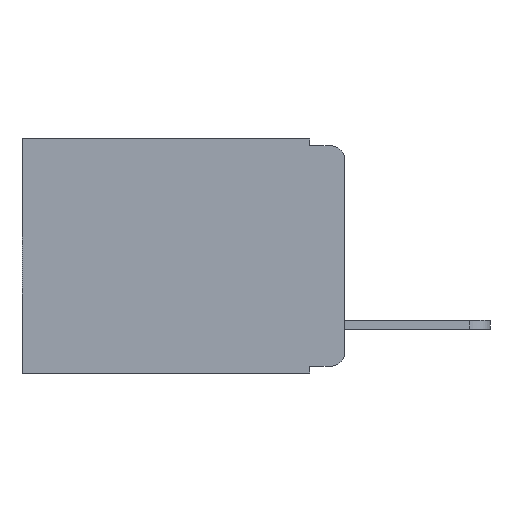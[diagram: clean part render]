
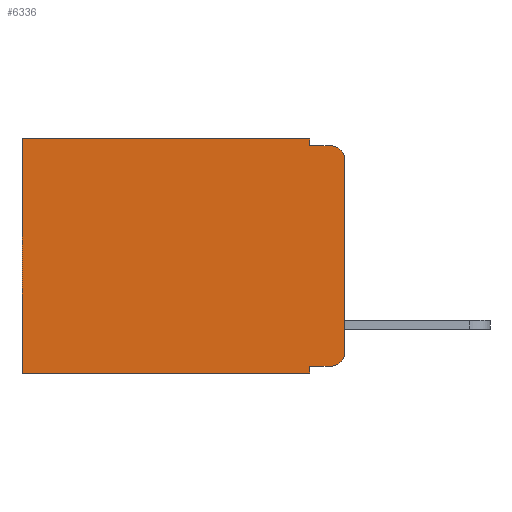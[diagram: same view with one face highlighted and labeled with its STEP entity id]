
A CAD part, left-side view. The second image highlights one B-rep face of the part: STEP entity #6336.
In plain terms, the highlighted planar face has unit normal (-1, 0, 0).
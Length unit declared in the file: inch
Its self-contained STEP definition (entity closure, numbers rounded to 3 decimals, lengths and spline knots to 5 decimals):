
#645 = DIRECTION ( 'NONE',  ( 1., 0., 0. ) ) ;
#750 = ORIENTED_EDGE ( 'NONE', *, *, #5122, .F. ) ;
#910 = EDGE_CURVE ( 'NONE', #9293, #7020, #4795, .T. ) ;
#1124 = CARTESIAN_POINT ( 'NONE',  ( 0.298, 0.051, -0.343 ) ) ;
#1326 = LINE ( 'NONE', #2875, #3736 ) ;
#1725 = ORIENTED_EDGE ( 'NONE', *, *, #4528, .T. ) ;
#1951 = VERTEX_POINT ( 'NONE', #9097 ) ;
#1993 = DIRECTION ( 'NONE',  ( -1., 0., 0. ) ) ;
#2035 = DIRECTION ( 'NONE',  ( -1., 0., 0. ) ) ;
#2044 = EDGE_CURVE ( 'NONE', #8071, #1951, #2216, .T. ) ;
#2069 = EDGE_CURVE ( 'NONE', #9875, #7020, #5048, .T. ) ;
#2093 = LINE ( 'NONE', #3935, #7123 ) ;
#2190 = ORIENTED_EDGE ( 'NONE', *, *, #4158, .F. ) ;
#2216 = LINE ( 'NONE', #5686, #4355 ) ;
#2301 = ORIENTED_EDGE ( 'NONE', *, *, #7854, .T. ) ;
#2359 = AXIS2_PLACEMENT_3D ( 'NONE', #6765, #645, #7810 ) ;
#2486 = CARTESIAN_POINT ( 'NONE',  ( 0.298, 0.473, -0.343 ) ) ;
#2571 = EDGE_CURVE ( 'NONE', #8071, #10523, #3902, .T. ) ;
#2668 = VECTOR ( 'NONE', #9058, 39.37008 ) ;
#2875 = CARTESIAN_POINT ( 'NONE',  ( 0.298, 0.051, 0. ) ) ;
#2957 = VERTEX_POINT ( 'NONE', #6184 ) ;
#2982 = AXIS2_PLACEMENT_3D ( 'NONE', #10907, #2035, #4866 ) ;
#3039 = DIRECTION ( 'NONE',  ( 0., 0., -1. ) ) ;
#3416 = DIRECTION ( 'NONE',  ( 0., 1., 0. ) ) ;
#3697 = EDGE_CURVE ( 'NONE', #2957, #9293, #9426, .T. ) ;
#3736 = VECTOR ( 'NONE', #9085, 39.37008 ) ;
#3887 = CARTESIAN_POINT ( 'NONE',  ( 0.298, 0.473, 0. ) ) ;
#3902 = CIRCLE ( 'NONE', #2982, 0.02 ) ;
#3903 = ORIENTED_EDGE ( 'NONE', *, *, #4371, .F. ) ;
#3935 = CARTESIAN_POINT ( 'NONE',  ( 0.298, 0.051, -0.333 ) ) ;
#3965 = CARTESIAN_POINT ( 'NONE',  ( 0.298, 0., -0.03 ) ) ;
#3972 = CARTESIAN_POINT ( 'NONE',  ( 0.298, 0.473, 0. ) ) ;
#4158 = EDGE_CURVE ( 'NONE', #11109, #9875, #1326, .T. ) ;
#4263 = AXIS2_PLACEMENT_3D ( 'NONE', #6547, #1993, #9215 ) ;
#4355 = VECTOR ( 'NONE', #3039, 39.37008 ) ;
#4371 = EDGE_CURVE ( 'NONE', #2957, #4569, #7675, .T. ) ;
#4528 = EDGE_CURVE ( 'NONE', #11109, #10031, #2093, .T. ) ;
#4562 = ORIENTED_EDGE ( 'NONE', *, *, #2044, .F. ) ;
#4569 = VERTEX_POINT ( 'NONE', #7809 ) ;
#4795 = LINE ( 'NONE', #3887, #2668 ) ;
#4866 = DIRECTION ( 'NONE',  ( 0., 0., -1. ) ) ;
#5048 = LINE ( 'NONE', #7493, #5734 ) ;
#5122 = EDGE_CURVE ( 'NONE', #4569, #10523, #5923, .T. ) ;
#5468 = ORIENTED_EDGE ( 'NONE', *, *, #3697, .T. ) ;
#5686 = CARTESIAN_POINT ( 'NONE',  ( 0.298, 0., 0. ) ) ;
#5715 = CARTESIAN_POINT ( 'NONE',  ( 0.298, 0.02, -0.01 ) ) ;
#5734 = VECTOR ( 'NONE', #7425, 39.37008 ) ;
#5923 = LINE ( 'NONE', #8517, #6875 ) ;
#6042 = PLANE ( 'NONE',  #2359 ) ;
#6054 = CARTESIAN_POINT ( 'NONE',  ( 0.298, 0., 0. ) ) ;
#6184 = CARTESIAN_POINT ( 'NONE',  ( 0.298, 0.051, 0. ) ) ;
#6336 = ADVANCED_FACE ( 'NONE', ( #6850 ), #6042, .F. ) ;
#6547 = CARTESIAN_POINT ( 'NONE',  ( 0.298, 0.02, -0.313 ) ) ;
#6622 = DIRECTION ( 'NONE',  ( 0., -1., 0. ) ) ;
#6765 = CARTESIAN_POINT ( 'NONE',  ( 0.298, 0., 0. ) ) ;
#6850 = FACE_OUTER_BOUND ( 'NONE', #7235, .T. ) ;
#6875 = VECTOR ( 'NONE', #9408, 39.37008 ) ;
#6990 = VECTOR ( 'NONE', #11486, 39.37008 ) ;
#7020 = VERTEX_POINT ( 'NONE', #2486 ) ;
#7123 = VECTOR ( 'NONE', #6622, 39.37008 ) ;
#7235 = EDGE_LOOP ( 'NONE', ( #4562, #9000, #750, #3903, #5468, #7436, #8824, #2190, #1725, #2301 ) ) ;
#7425 = DIRECTION ( 'NONE',  ( 0., 1., 0. ) ) ;
#7436 = ORIENTED_EDGE ( 'NONE', *, *, #910, .T. ) ;
#7493 = CARTESIAN_POINT ( 'NONE',  ( 0.298, 0., -0.343 ) ) ;
#7675 = LINE ( 'NONE', #8848, #6990 ) ;
#7809 = CARTESIAN_POINT ( 'NONE',  ( 0.298, 0.051, -0.01 ) ) ;
#7810 = DIRECTION ( 'NONE',  ( 0., 0., -1. ) ) ;
#7854 = EDGE_CURVE ( 'NONE', #10031, #1951, #11334, .T. ) ;
#8071 = VERTEX_POINT ( 'NONE', #3965 ) ;
#8517 = CARTESIAN_POINT ( 'NONE',  ( 0.298, 0.051, -0.01 ) ) ;
#8824 = ORIENTED_EDGE ( 'NONE', *, *, #2069, .F. ) ;
#8848 = CARTESIAN_POINT ( 'NONE',  ( 0.298, 0.051, 0. ) ) ;
#9000 = ORIENTED_EDGE ( 'NONE', *, *, #2571, .T. ) ;
#9058 = DIRECTION ( 'NONE',  ( 0., 0., -1. ) ) ;
#9085 = DIRECTION ( 'NONE',  ( 0., 0., -1. ) ) ;
#9097 = CARTESIAN_POINT ( 'NONE',  ( 0.298, 0., -0.313 ) ) ;
#9215 = DIRECTION ( 'NONE',  ( 0., 0., -1. ) ) ;
#9293 = VERTEX_POINT ( 'NONE', #3972 ) ;
#9383 = CARTESIAN_POINT ( 'NONE',  ( 0.298, 0.051, -0.333 ) ) ;
#9408 = DIRECTION ( 'NONE',  ( 0., -1., 0. ) ) ;
#9426 = LINE ( 'NONE', #6054, #9723 ) ;
#9723 = VECTOR ( 'NONE', #3416, 39.37008 ) ;
#9875 = VERTEX_POINT ( 'NONE', #1124 ) ;
#10031 = VERTEX_POINT ( 'NONE', #11227 ) ;
#10523 = VERTEX_POINT ( 'NONE', #5715 ) ;
#10907 = CARTESIAN_POINT ( 'NONE',  ( 0.298, 0.02, -0.03 ) ) ;
#11109 = VERTEX_POINT ( 'NONE', #9383 ) ;
#11227 = CARTESIAN_POINT ( 'NONE',  ( 0.298, 0.02, -0.333 ) ) ;
#11334 = CIRCLE ( 'NONE', #4263, 0.02 ) ;
#11486 = DIRECTION ( 'NONE',  ( 0., 0., -1. ) ) ;
